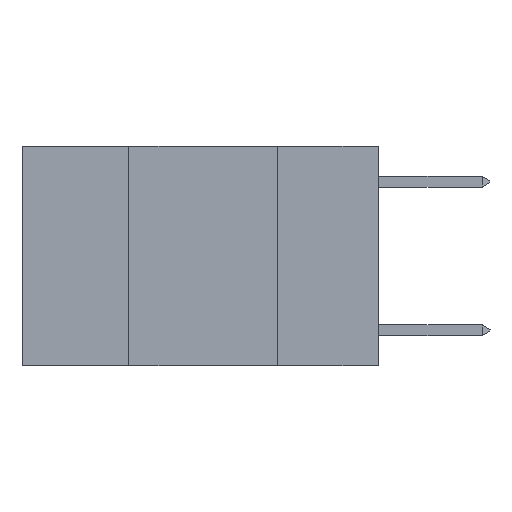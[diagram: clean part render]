
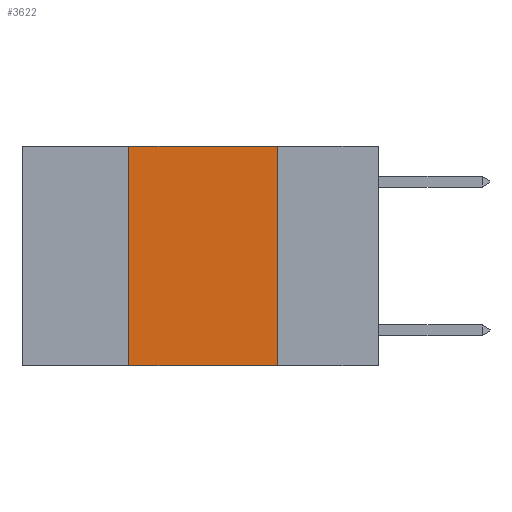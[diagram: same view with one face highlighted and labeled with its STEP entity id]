
A CAD part, left-side view. The second image highlights one B-rep face of the part: STEP entity #3622.
In plain terms, the highlighted planar face has unit normal (-1, 0, 0).
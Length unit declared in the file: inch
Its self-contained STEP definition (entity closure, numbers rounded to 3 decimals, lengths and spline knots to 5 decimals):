
#363 = DIRECTION ( 'NONE',  ( 0., 0., -1. ) ) ;
#571 = EDGE_CURVE ( 'NONE', #6078, #11510, #10825, .T. ) ;
#593 = ORIENTED_EDGE ( 'NONE', *, *, #571, .F. ) ;
#1492 = ORIENTED_EDGE ( 'NONE', *, *, #16819, .F. ) ;
#1614 = VECTOR ( 'NONE', #16663, 39.37008 ) ;
#1940 = ORIENTED_EDGE ( 'NONE', *, *, #16494, .T. ) ;
#2290 = DIRECTION ( 'NONE',  ( 0., -1., 0. ) ) ;
#3567 = CARTESIAN_POINT ( 'NONE',  ( 0., 0.17, 0. ) ) ;
#3622 = ADVANCED_FACE ( 'NONE', ( #12585 ), #13495, .F. ) ;
#3698 = VECTOR ( 'NONE', #2290, 39.37008 ) ;
#5087 = CARTESIAN_POINT ( 'NONE',  ( 0., 0.17, -0.37 ) ) ;
#5336 = VECTOR ( 'NONE', #10027, 39.37008 ) ;
#5532 = LINE ( 'NONE', #6422, #1614 ) ;
#5658 = DIRECTION ( 'NONE',  ( 1., 0., 0. ) ) ;
#6078 = VERTEX_POINT ( 'NONE', #16774 ) ;
#6422 = CARTESIAN_POINT ( 'NONE',  ( 0., 0.42, 0. ) ) ;
#7240 = VECTOR ( 'NONE', #363, 39.37008 ) ;
#7554 = CARTESIAN_POINT ( 'NONE',  ( 0., 0.17, 0. ) ) ;
#8653 = VERTEX_POINT ( 'NONE', #5087 ) ;
#8748 = CARTESIAN_POINT ( 'NONE',  ( 0., 0.6, -0.37 ) ) ;
#9301 = VERTEX_POINT ( 'NONE', #16415 ) ;
#9619 = CARTESIAN_POINT ( 'NONE',  ( 0., 0.6, 0. ) ) ;
#9698 = LINE ( 'NONE', #8748, #5336 ) ;
#10027 = DIRECTION ( 'NONE',  ( 0., -1., 0. ) ) ;
#10736 = LINE ( 'NONE', #7554, #7240 ) ;
#10825 = LINE ( 'NONE', #13888, #3698 ) ;
#11510 = VERTEX_POINT ( 'NONE', #3567 ) ;
#12585 = FACE_OUTER_BOUND ( 'NONE', #13105, .T. ) ;
#13105 = EDGE_LOOP ( 'NONE', ( #14929, #593, #1492, #1940 ) ) ;
#13271 = AXIS2_PLACEMENT_3D ( 'NONE', #9619, #5658, #14730 ) ;
#13495 = PLANE ( 'NONE',  #13271 ) ;
#13888 = CARTESIAN_POINT ( 'NONE',  ( 0., 0.6, 0. ) ) ;
#14144 = EDGE_CURVE ( 'NONE', #11510, #8653, #10736, .T. ) ;
#14730 = DIRECTION ( 'NONE',  ( 0., 0., -1. ) ) ;
#14929 = ORIENTED_EDGE ( 'NONE', *, *, #14144, .F. ) ;
#16415 = CARTESIAN_POINT ( 'NONE',  ( 0., 0.42, -0.37 ) ) ;
#16494 = EDGE_CURVE ( 'NONE', #9301, #8653, #9698, .T. ) ;
#16663 = DIRECTION ( 'NONE',  ( 0., 0., 1. ) ) ;
#16774 = CARTESIAN_POINT ( 'NONE',  ( 0., 0.42, 0. ) ) ;
#16819 = EDGE_CURVE ( 'NONE', #9301, #6078, #5532, .T. ) ;
